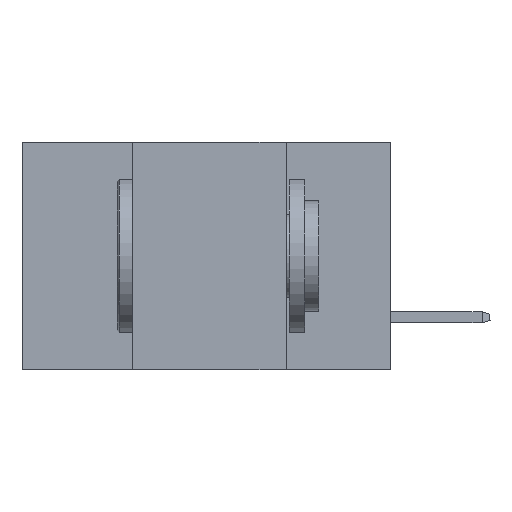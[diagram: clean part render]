
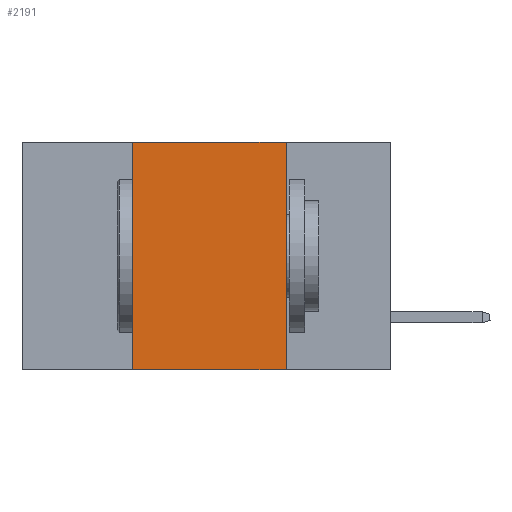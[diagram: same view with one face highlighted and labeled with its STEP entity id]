
A CAD part, left-side view. The second image highlights one B-rep face of the part: STEP entity #2191.
In plain terms, the highlighted planar face has unit normal (-1, 0, 0).
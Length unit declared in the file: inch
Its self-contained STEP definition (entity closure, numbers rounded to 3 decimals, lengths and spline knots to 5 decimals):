
#385 = FACE_OUTER_BOUND ( 'NONE', #9729, .T. ) ;
#469 = LINE ( 'NONE', #4066, #7298 ) ;
#593 = ORIENTED_EDGE ( 'NONE', *, *, #4625, .F. ) ;
#980 = VERTEX_POINT ( 'NONE', #6273 ) ;
#1542 = CARTESIAN_POINT ( 'NONE',  ( 0., 0.6, 0. ) ) ;
#1547 = VERTEX_POINT ( 'NONE', #6464 ) ;
#1570 = EDGE_CURVE ( 'NONE', #5627, #8901, #1899, .T. ) ;
#1899 = LINE ( 'NONE', #5309, #3023 ) ;
#2191 = ADVANCED_FACE ( 'NONE', ( #385 ), #4980, .F. ) ;
#2852 = DIRECTION ( 'NONE',  ( 1., 0., 0. ) ) ;
#2915 = CARTESIAN_POINT ( 'NONE',  ( 0., 0.42, -0.37 ) ) ;
#3023 = VECTOR ( 'NONE', #3837, 39.37008 ) ;
#3644 = ORIENTED_EDGE ( 'NONE', *, *, #4666, .T. ) ;
#3837 = DIRECTION ( 'NONE',  ( 0., 0., 1. ) ) ;
#3929 = VECTOR ( 'NONE', #10076, 39.37008 ) ;
#4028 = DIRECTION ( 'NONE',  ( 0., -1., 0. ) ) ;
#4066 = CARTESIAN_POINT ( 'NONE',  ( 0., 0.6, -0.37 ) ) ;
#4116 = ORIENTED_EDGE ( 'NONE', *, *, #1570, .F. ) ;
#4625 = EDGE_CURVE ( 'NONE', #980, #1547, #4963, .T. ) ;
#4666 = EDGE_CURVE ( 'NONE', #5627, #1547, #469, .T. ) ;
#4757 = AXIS2_PLACEMENT_3D ( 'NONE', #5947, #2852, #7519 ) ;
#4963 = LINE ( 'NONE', #9347, #9378 ) ;
#4980 = PLANE ( 'NONE',  #4757 ) ;
#5309 = CARTESIAN_POINT ( 'NONE',  ( 0., 0.42, 0. ) ) ;
#5627 = VERTEX_POINT ( 'NONE', #2915 ) ;
#5947 = CARTESIAN_POINT ( 'NONE',  ( 0., 0.6, 0. ) ) ;
#6273 = CARTESIAN_POINT ( 'NONE',  ( 0., 0.17, 0. ) ) ;
#6464 = CARTESIAN_POINT ( 'NONE',  ( 0., 0.17, -0.37 ) ) ;
#7007 = DIRECTION ( 'NONE',  ( 0., 0., -1. ) ) ;
#7039 = EDGE_CURVE ( 'NONE', #8901, #980, #7739, .T. ) ;
#7298 = VECTOR ( 'NONE', #4028, 39.37008 ) ;
#7519 = DIRECTION ( 'NONE',  ( 0., 0., -1. ) ) ;
#7673 = CARTESIAN_POINT ( 'NONE',  ( 0., 0.42, 0. ) ) ;
#7739 = LINE ( 'NONE', #1542, #3929 ) ;
#8824 = ORIENTED_EDGE ( 'NONE', *, *, #7039, .F. ) ;
#8901 = VERTEX_POINT ( 'NONE', #7673 ) ;
#9347 = CARTESIAN_POINT ( 'NONE',  ( 0., 0.17, 0. ) ) ;
#9378 = VECTOR ( 'NONE', #7007, 39.37008 ) ;
#9729 = EDGE_LOOP ( 'NONE', ( #593, #8824, #4116, #3644 ) ) ;
#10076 = DIRECTION ( 'NONE',  ( 0., -1., 0. ) ) ;
